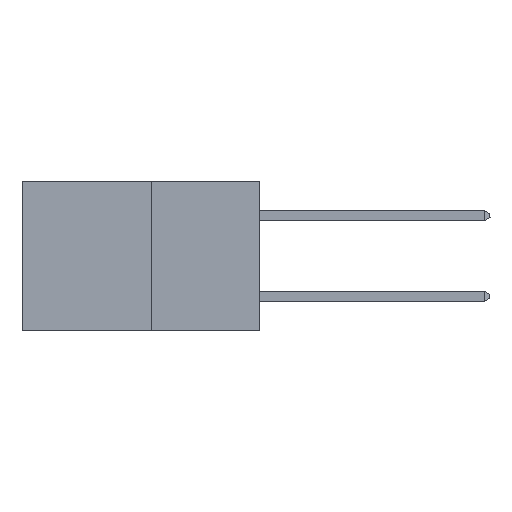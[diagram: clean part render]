
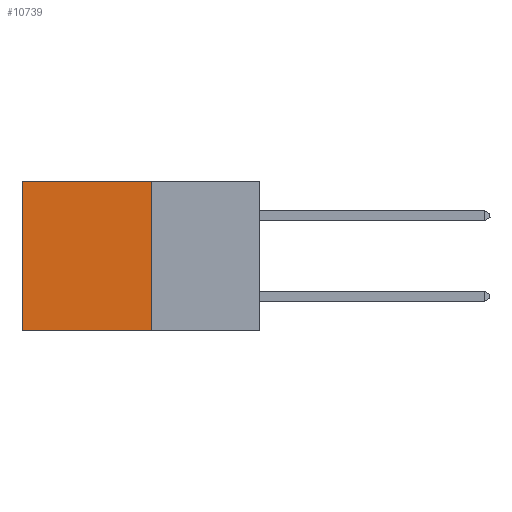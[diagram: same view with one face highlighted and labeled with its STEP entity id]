
A CAD part, left-side view. The second image highlights one B-rep face of the part: STEP entity #10739.
In plain terms, the highlighted planar face has unit normal (-1, 0, 0).
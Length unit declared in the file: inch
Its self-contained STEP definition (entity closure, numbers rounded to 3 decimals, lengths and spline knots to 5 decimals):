
#866 = EDGE_CURVE ( 'NONE', #2437, #26557, #18941, .T. ) ;
#959 = LINE ( 'NONE', #1585, #16389 ) ;
#974 = EDGE_CURVE ( 'NONE', #2437, #8030, #959, .T. ) ;
#1585 = CARTESIAN_POINT ( 'NONE',  ( 0.277, 0.27, 0. ) ) ;
#1867 = DIRECTION ( 'NONE',  ( 0., 0., -1. ) ) ;
#2064 = DIRECTION ( 'NONE',  ( 0., 1., 0. ) ) ;
#2158 = CARTESIAN_POINT ( 'NONE',  ( 0.277, 0.27, -0.37 ) ) ;
#2424 = DIRECTION ( 'NONE',  ( 0., 0., -1. ) ) ;
#2437 = VERTEX_POINT ( 'NONE', #4948 ) ;
#3737 = EDGE_CURVE ( 'NONE', #8030, #14180, #10760, .T. ) ;
#4948 = CARTESIAN_POINT ( 'NONE',  ( 0.277, 0.27, 0. ) ) ;
#5610 = EDGE_LOOP ( 'NONE', ( #22783, #7560, #25655, #24083 ) ) ;
#6440 = CARTESIAN_POINT ( 'NONE',  ( 0.277, 0.59, -0.37 ) ) ;
#6951 = PLANE ( 'NONE',  #17059 ) ;
#7560 = ORIENTED_EDGE ( 'NONE', *, *, #16911, .F. ) ;
#7962 = VECTOR ( 'NONE', #2424, 39.37008 ) ;
#8030 = VERTEX_POINT ( 'NONE', #17985 ) ;
#8087 = CARTESIAN_POINT ( 'NONE',  ( 0.277, 0.27, -0.37 ) ) ;
#8246 = FACE_OUTER_BOUND ( 'NONE', #5610, .T. ) ;
#8380 = CARTESIAN_POINT ( 'NONE',  ( 0.277, 0.59, -0.37 ) ) ;
#9083 = DIRECTION ( 'NONE',  ( 1., 0., 0. ) ) ;
#10114 = VECTOR ( 'NONE', #1867, 39.37008 ) ;
#10739 = ADVANCED_FACE ( 'NONE', ( #8246 ), #6951, .F. ) ;
#10760 = LINE ( 'NONE', #6440, #10114 ) ;
#12848 = LINE ( 'NONE', #8087, #23150 ) ;
#12939 = CARTESIAN_POINT ( 'NONE',  ( 0.277, 0.27, -0.37 ) ) ;
#14180 = VERTEX_POINT ( 'NONE', #8380 ) ;
#16389 = VECTOR ( 'NONE', #2064, 39.37008 ) ;
#16911 = EDGE_CURVE ( 'NONE', #26557, #14180, #12848, .T. ) ;
#17059 = AXIS2_PLACEMENT_3D ( 'NONE', #17284, #9083, #23523 ) ;
#17284 = CARTESIAN_POINT ( 'NONE',  ( 0.277, 0.27, -0.37 ) ) ;
#17985 = CARTESIAN_POINT ( 'NONE',  ( 0.277, 0.59, 0. ) ) ;
#18941 = LINE ( 'NONE', #2158, #7962 ) ;
#22783 = ORIENTED_EDGE ( 'NONE', *, *, #3737, .T. ) ;
#23150 = VECTOR ( 'NONE', #26626, 39.37008 ) ;
#23523 = DIRECTION ( 'NONE',  ( 0., 0., -1. ) ) ;
#24083 = ORIENTED_EDGE ( 'NONE', *, *, #974, .T. ) ;
#25655 = ORIENTED_EDGE ( 'NONE', *, *, #866, .F. ) ;
#26557 = VERTEX_POINT ( 'NONE', #12939 ) ;
#26626 = DIRECTION ( 'NONE',  ( 0., 1., 0. ) ) ;
